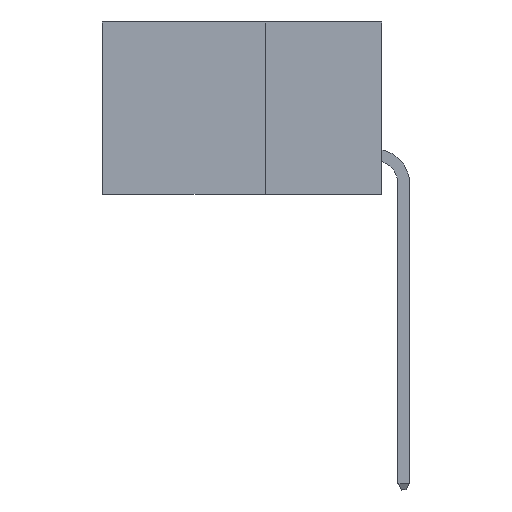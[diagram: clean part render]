
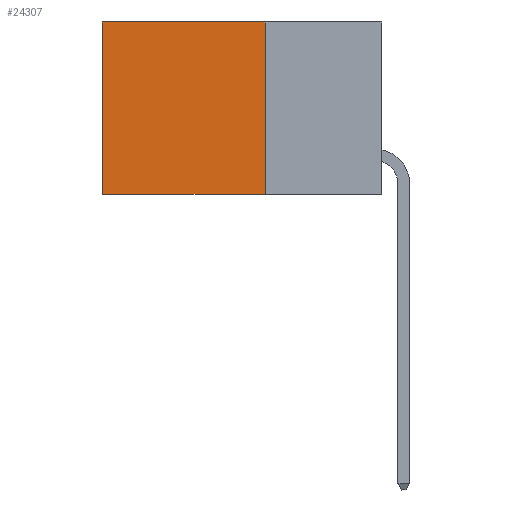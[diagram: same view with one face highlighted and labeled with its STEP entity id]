
A CAD part, left-side view. The second image highlights one B-rep face of the part: STEP entity #24307.
In plain terms, the highlighted planar face has unit normal (-1, 0, 0).
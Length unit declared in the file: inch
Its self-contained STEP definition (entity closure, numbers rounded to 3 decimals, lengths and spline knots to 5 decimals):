
#768 = PLANE ( 'NONE',  #4505 ) ;
#3764 = CARTESIAN_POINT ( 'NONE',  ( 0.2875, 0.25, 0. ) ) ;
#4073 = VERTEX_POINT ( 'NONE', #11106 ) ;
#4295 = DIRECTION ( 'NONE',  ( 0., 1., 0. ) ) ;
#4505 = AXIS2_PLACEMENT_3D ( 'NONE', #3764, #9330, #23537 ) ;
#5799 = DIRECTION ( 'NONE',  ( 0., 1., 0. ) ) ;
#8965 = LINE ( 'NONE', #9544, #11160 ) ;
#9330 = DIRECTION ( 'NONE',  ( 1., 0., 0. ) ) ;
#9544 = CARTESIAN_POINT ( 'NONE',  ( 0.2875, 0.25, 0. ) ) ;
#9918 = EDGE_CURVE ( 'NONE', #4073, #19816, #8965, .T. ) ;
#10795 = VERTEX_POINT ( 'NONE', #36220 ) ;
#11106 = CARTESIAN_POINT ( 'NONE',  ( 0.2875, 0.25, 0. ) ) ;
#11160 = VECTOR ( 'NONE', #14858, 39.37008 ) ;
#12856 = LINE ( 'NONE', #34432, #27438 ) ;
#13332 = EDGE_CURVE ( 'NONE', #19816, #23155, #12856, .T. ) ;
#14646 = CARTESIAN_POINT ( 'NONE',  ( 0.2875, 0.6, -0.37 ) ) ;
#14858 = DIRECTION ( 'NONE',  ( 0., 0., -1. ) ) ;
#18223 = CARTESIAN_POINT ( 'NONE',  ( 0.2875, 0.25, -0.37 ) ) ;
#18787 = ORIENTED_EDGE ( 'NONE', *, *, #34629, .T. ) ;
#19655 = VECTOR ( 'NONE', #30710, 39.37008 ) ;
#19816 = VERTEX_POINT ( 'NONE', #18223 ) ;
#23155 = VERTEX_POINT ( 'NONE', #14646 ) ;
#23537 = DIRECTION ( 'NONE',  ( 0., 0., -1. ) ) ;
#23943 = CARTESIAN_POINT ( 'NONE',  ( 0.2875, 0.25, 0. ) ) ;
#24027 = EDGE_CURVE ( 'NONE', #10795, #23155, #25401, .T. ) ;
#24307 = ADVANCED_FACE ( 'NONE', ( #26699 ), #768, .F. ) ;
#24584 = LINE ( 'NONE', #23943, #33428 ) ;
#25401 = LINE ( 'NONE', #33430, #19655 ) ;
#26699 = FACE_OUTER_BOUND ( 'NONE', #30344, .T. ) ;
#27438 = VECTOR ( 'NONE', #5799, 39.37008 ) ;
#28852 = ORIENTED_EDGE ( 'NONE', *, *, #24027, .T. ) ;
#28941 = ORIENTED_EDGE ( 'NONE', *, *, #13332, .F. ) ;
#30344 = EDGE_LOOP ( 'NONE', ( #28852, #28941, #36520, #18787 ) ) ;
#30710 = DIRECTION ( 'NONE',  ( 0., 0., -1. ) ) ;
#33428 = VECTOR ( 'NONE', #4295, 39.37008 ) ;
#33430 = CARTESIAN_POINT ( 'NONE',  ( 0.2875, 0.6, 0. ) ) ;
#34432 = CARTESIAN_POINT ( 'NONE',  ( 0.2875, 0.25, -0.37 ) ) ;
#34629 = EDGE_CURVE ( 'NONE', #4073, #10795, #24584, .T. ) ;
#36220 = CARTESIAN_POINT ( 'NONE',  ( 0.2875, 0.6, 0. ) ) ;
#36520 = ORIENTED_EDGE ( 'NONE', *, *, #9918, .F. ) ;
